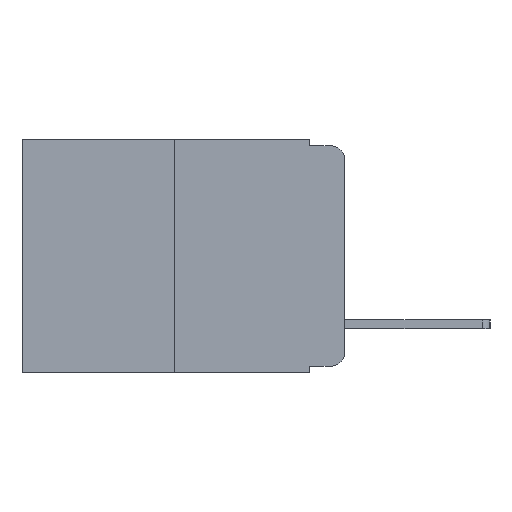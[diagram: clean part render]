
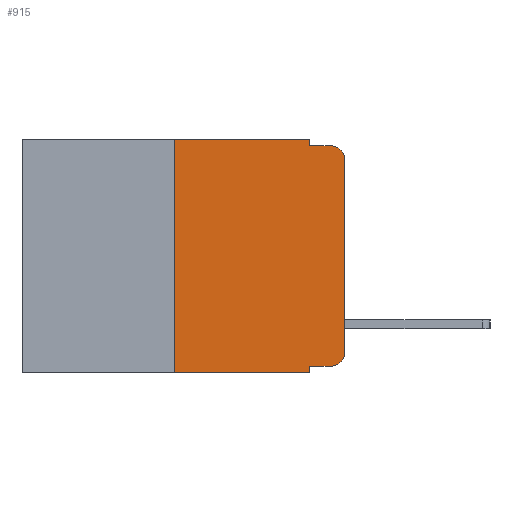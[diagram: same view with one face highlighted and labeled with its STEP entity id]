
A CAD part, left-side view. The second image highlights one B-rep face of the part: STEP entity #915.
In plain terms, the highlighted planar face has unit normal (-1, 0, 0).
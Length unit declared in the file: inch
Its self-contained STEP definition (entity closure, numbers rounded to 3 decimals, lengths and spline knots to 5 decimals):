
#22 = ORIENTED_EDGE ( 'NONE', *, *, #5557, .F. ) ;
#126 = ORIENTED_EDGE ( 'NONE', *, *, #4671, .T. ) ;
#284 = ORIENTED_EDGE ( 'NONE', *, *, #4417, .F. ) ;
#335 = ORIENTED_EDGE ( 'NONE', *, *, #7509, .T. ) ;
#404 = VERTEX_POINT ( 'NONE', #5185 ) ;
#455 = ORIENTED_EDGE ( 'NONE', *, *, #8808, .F. ) ;
#506 = ORIENTED_EDGE ( 'NONE', *, *, #3605, .F. ) ;
#515 = VERTEX_POINT ( 'NONE', #5730 ) ;
#839 = ORIENTED_EDGE ( 'NONE', *, *, #1744, .T. ) ;
#915 = ADVANCED_FACE ( 'NONE', ( #3450 ), #3437, .F. ) ;
#952 = ORIENTED_EDGE ( 'NONE', *, *, #7788, .T. ) ;
#1125 = EDGE_LOOP ( 'NONE', ( #7465, #126, #455, #284, #5321, #22, #335, #506, #839, #952 ) ) ;
#1237 = CARTESIAN_POINT ( 'NONE',  ( 0., 0., 0. ) ) ;
#1293 = LINE ( 'NONE', #1672, #5950 ) ;
#1659 = LINE ( 'NONE', #10220, #8391 ) ;
#1672 = CARTESIAN_POINT ( 'NONE',  ( 0., 0.473, 0. ) ) ;
#1744 = EDGE_CURVE ( 'NONE', #8750, #6811, #6848, .T. ) ;
#2191 = VECTOR ( 'NONE', #2231, 39.37008 ) ;
#2231 = DIRECTION ( 'NONE',  ( 0., 0., 1. ) ) ;
#2335 = CARTESIAN_POINT ( 'NONE',  ( 0., 0.25, 0. ) ) ;
#2434 = VECTOR ( 'NONE', #8192, 39.37008 ) ;
#2606 = VERTEX_POINT ( 'NONE', #3231 ) ;
#2675 = CARTESIAN_POINT ( 'NONE',  ( 0., 0.02, -0.333 ) ) ;
#2697 = CARTESIAN_POINT ( 'NONE',  ( 0., 0.051, -0.01 ) ) ;
#3097 = CARTESIAN_POINT ( 'NONE',  ( 0., 0.051, 0. ) ) ;
#3231 = CARTESIAN_POINT ( 'NONE',  ( 0., 0.25, -0.343 ) ) ;
#3386 = DIRECTION ( 'NONE',  ( -1., 0., 0. ) ) ;
#3437 = PLANE ( 'NONE',  #4834 ) ;
#3450 = FACE_OUTER_BOUND ( 'NONE', #1125, .T. ) ;
#3605 = EDGE_CURVE ( 'NONE', #8750, #9587, #11161, .T. ) ;
#3775 = CARTESIAN_POINT ( 'NONE',  ( 0., 0.051, -0.333 ) ) ;
#4215 = DIRECTION ( 'NONE',  ( 0., -1., 0. ) ) ;
#4417 = EDGE_CURVE ( 'NONE', #8546, #5075, #9157, .T. ) ;
#4553 = CARTESIAN_POINT ( 'NONE',  ( 0., 0.02, -0.01 ) ) ;
#4592 = CARTESIAN_POINT ( 'NONE',  ( 0., 0.051, -0.343 ) ) ;
#4671 = EDGE_CURVE ( 'NONE', #515, #7486, #5724, .T. ) ;
#4834 = AXIS2_PLACEMENT_3D ( 'NONE', #7548, #9094, #9083 ) ;
#5075 = VERTEX_POINT ( 'NONE', #2697 ) ;
#5151 = CARTESIAN_POINT ( 'NONE',  ( 0., 0.051, -0.01 ) ) ;
#5185 = CARTESIAN_POINT ( 'NONE',  ( 0., 0., -0.313 ) ) ;
#5321 = ORIENTED_EDGE ( 'NONE', *, *, #9618, .F. ) ;
#5557 = EDGE_CURVE ( 'NONE', #2606, #7882, #11252, .T. ) ;
#5582 = VECTOR ( 'NONE', #5953, 39.37008 ) ;
#5628 = CARTESIAN_POINT ( 'NONE',  ( 0., 0.02, -0.313 ) ) ;
#5724 = CIRCLE ( 'NONE', #7816, 0.02 ) ;
#5730 = CARTESIAN_POINT ( 'NONE',  ( 0., 0., -0.03 ) ) ;
#5950 = VECTOR ( 'NONE', #10250, 39.37008 ) ;
#5953 = DIRECTION ( 'NONE',  ( 0., -1., 0. ) ) ;
#6342 = CIRCLE ( 'NONE', #9945, 0.02 ) ;
#6407 = DIRECTION ( 'NONE',  ( 0., 0., -1. ) ) ;
#6475 = CARTESIAN_POINT ( 'NONE',  ( 0., 0.25, 0. ) ) ;
#6589 = DIRECTION ( 'NONE',  ( 0., 0., -1. ) ) ;
#6811 = VERTEX_POINT ( 'NONE', #2675 ) ;
#6848 = LINE ( 'NONE', #3775, #9288 ) ;
#6959 = VECTOR ( 'NONE', #6589, 39.37008 ) ;
#7465 = ORIENTED_EDGE ( 'NONE', *, *, #10814, .T. ) ;
#7476 = CARTESIAN_POINT ( 'NONE',  ( 0., 0.051, -0.333 ) ) ;
#7486 = VERTEX_POINT ( 'NONE', #4553 ) ;
#7509 = EDGE_CURVE ( 'NONE', #2606, #9587, #1659, .T. ) ;
#7548 = CARTESIAN_POINT ( 'NONE',  ( 0., 0.473, 0. ) ) ;
#7788 = EDGE_CURVE ( 'NONE', #6811, #404, #6342, .T. ) ;
#7816 = AXIS2_PLACEMENT_3D ( 'NONE', #8420, #3386, #9243 ) ;
#7882 = VERTEX_POINT ( 'NONE', #6475 ) ;
#8192 = DIRECTION ( 'NONE',  ( 0., 0., -1. ) ) ;
#8391 = VECTOR ( 'NONE', #10995, 39.37008 ) ;
#8420 = CARTESIAN_POINT ( 'NONE',  ( 0., 0.02, -0.03 ) ) ;
#8546 = VERTEX_POINT ( 'NONE', #8781 ) ;
#8750 = VERTEX_POINT ( 'NONE', #7476 ) ;
#8781 = CARTESIAN_POINT ( 'NONE',  ( 0., 0.051, 0. ) ) ;
#8808 = EDGE_CURVE ( 'NONE', #5075, #7486, #9891, .T. ) ;
#9083 = DIRECTION ( 'NONE',  ( 0., 0., -1. ) ) ;
#9094 = DIRECTION ( 'NONE',  ( 1., 0., 0. ) ) ;
#9109 = LINE ( 'NONE', #1237, #2191 ) ;
#9157 = LINE ( 'NONE', #9851, #6959 ) ;
#9243 = DIRECTION ( 'NONE',  ( 0., 0., -1. ) ) ;
#9288 = VECTOR ( 'NONE', #4215, 39.37008 ) ;
#9587 = VERTEX_POINT ( 'NONE', #4592 ) ;
#9618 = EDGE_CURVE ( 'NONE', #7882, #8546, #1293, .T. ) ;
#9851 = CARTESIAN_POINT ( 'NONE',  ( 0., 0.051, 0. ) ) ;
#9891 = LINE ( 'NONE', #5151, #5582 ) ;
#9945 = AXIS2_PLACEMENT_3D ( 'NONE', #5628, #11238, #6407 ) ;
#10220 = CARTESIAN_POINT ( 'NONE',  ( 0., 0.473, -0.343 ) ) ;
#10250 = DIRECTION ( 'NONE',  ( 0., -1., 0. ) ) ;
#10811 = DIRECTION ( 'NONE',  ( 0., 0., 1. ) ) ;
#10814 = EDGE_CURVE ( 'NONE', #404, #515, #9109, .T. ) ;
#10995 = DIRECTION ( 'NONE',  ( 0., -1., 0. ) ) ;
#10997 = VECTOR ( 'NONE', #10811, 39.37008 ) ;
#11161 = LINE ( 'NONE', #3097, #2434 ) ;
#11238 = DIRECTION ( 'NONE',  ( -1., 0., 0. ) ) ;
#11252 = LINE ( 'NONE', #2335, #10997 ) ;
